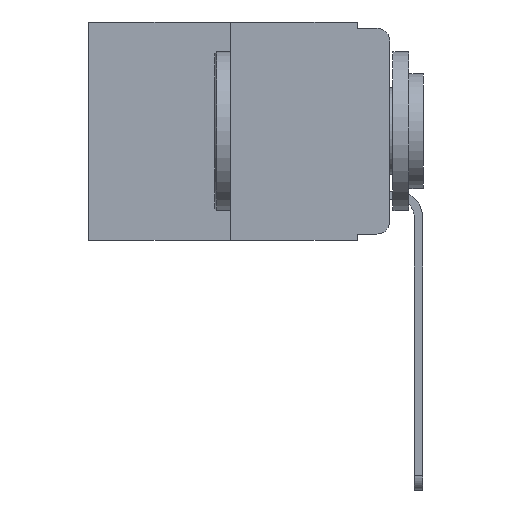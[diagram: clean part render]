
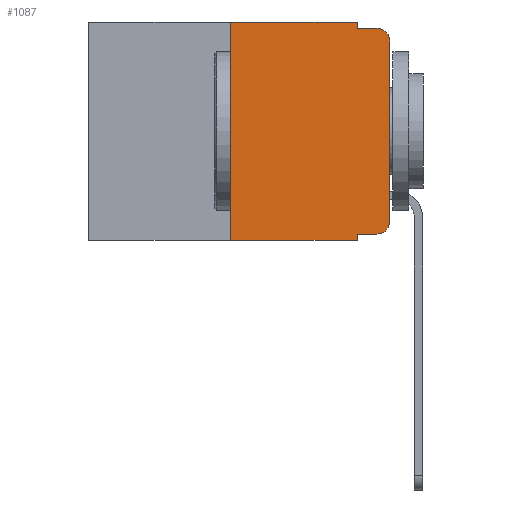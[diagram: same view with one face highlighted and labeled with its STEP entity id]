
A CAD part, left-side view. The second image highlights one B-rep face of the part: STEP entity #1087.
In plain terms, the highlighted planar face has unit normal (-1, 0, 0).
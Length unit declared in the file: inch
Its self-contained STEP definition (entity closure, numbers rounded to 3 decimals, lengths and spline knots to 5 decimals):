
#25 = VERTEX_POINT ( 'NONE', #7749 ) ;
#198 = ORIENTED_EDGE ( 'NONE', *, *, #9880, .T. ) ;
#398 = VERTEX_POINT ( 'NONE', #7649 ) ;
#482 = EDGE_CURVE ( 'NONE', #6446, #1942, #6358, .T. ) ;
#495 = DIRECTION ( 'NONE',  ( 0., -1., 0. ) ) ;
#609 = DIRECTION ( 'NONE',  ( 0., 0., 1. ) ) ;
#621 = AXIS2_PLACEMENT_3D ( 'NONE', #8059, #11972, #12167 ) ;
#648 = VERTEX_POINT ( 'NONE', #6341 ) ;
#877 = ORIENTED_EDGE ( 'NONE', *, *, #10707, .F. ) ;
#1087 = ADVANCED_FACE ( 'NONE', ( #11623 ), #9713, .F. ) ;
#1224 = DIRECTION ( 'NONE',  ( -1., 0., 0. ) ) ;
#1232 = VERTEX_POINT ( 'NONE', #9295 ) ;
#1382 = VECTOR ( 'NONE', #11126, 39.37008 ) ;
#1524 = EDGE_LOOP ( 'NONE', ( #8616, #7306, #877, #11440, #6873, #10229, #10753, #10109, #198, #8325 ) ) ;
#1886 = VECTOR ( 'NONE', #7356, 39.37008 ) ;
#1942 = VERTEX_POINT ( 'NONE', #2944 ) ;
#2054 = VERTEX_POINT ( 'NONE', #10558 ) ;
#2088 = EDGE_CURVE ( 'NONE', #7814, #1232, #7029, .T. ) ;
#2227 = CARTESIAN_POINT ( 'NONE',  ( 0., 0.051, 0. ) ) ;
#2288 = CARTESIAN_POINT ( 'NONE',  ( 0., 0.25, 0. ) ) ;
#2368 = LINE ( 'NONE', #2288, #9553 ) ;
#2627 = VERTEX_POINT ( 'NONE', #10738 ) ;
#2803 = DIRECTION ( 'NONE',  ( 0., -1., 0. ) ) ;
#2851 = VECTOR ( 'NONE', #4229, 39.37008 ) ;
#2944 = CARTESIAN_POINT ( 'NONE',  ( 0., 0.051, -0.343 ) ) ;
#3024 = EDGE_CURVE ( 'NONE', #2054, #25, #5633, .T. ) ;
#3972 = EDGE_CURVE ( 'NONE', #1232, #648, #7456, .T. ) ;
#4229 = DIRECTION ( 'NONE',  ( 0., 0., -1. ) ) ;
#4371 = CARTESIAN_POINT ( 'NONE',  ( 0., 0.02, -0.333 ) ) ;
#4451 = DIRECTION ( 'NONE',  ( -1., 0., 0. ) ) ;
#4474 = CARTESIAN_POINT ( 'NONE',  ( 0., 0.02, -0.313 ) ) ;
#4587 = EDGE_CURVE ( 'NONE', #398, #2054, #8627, .T. ) ;
#4700 = CARTESIAN_POINT ( 'NONE',  ( 0., 0.051, -0.01 ) ) ;
#5633 = LINE ( 'NONE', #2227, #2851 ) ;
#6057 = VECTOR ( 'NONE', #495, 39.37008 ) ;
#6341 = CARTESIAN_POINT ( 'NONE',  ( 0., 0., -0.03 ) ) ;
#6358 = LINE ( 'NONE', #11688, #6057 ) ;
#6428 = CARTESIAN_POINT ( 'NONE',  ( 0., 0.051, -0.333 ) ) ;
#6446 = VERTEX_POINT ( 'NONE', #8092 ) ;
#6471 = DIRECTION ( 'NONE',  ( 0., 0., -1. ) ) ;
#6512 = CARTESIAN_POINT ( 'NONE',  ( 0., 0.473, 0. ) ) ;
#6873 = ORIENTED_EDGE ( 'NONE', *, *, #4587, .F. ) ;
#6930 = CARTESIAN_POINT ( 'NONE',  ( 0., 0.02, -0.03 ) ) ;
#7029 = CIRCLE ( 'NONE', #8880, 0.02 ) ;
#7306 = ORIENTED_EDGE ( 'NONE', *, *, #8290, .T. ) ;
#7356 = DIRECTION ( 'NONE',  ( 0., -1., 0. ) ) ;
#7456 = LINE ( 'NONE', #10349, #9958 ) ;
#7649 = CARTESIAN_POINT ( 'NONE',  ( 0., 0.25, 0. ) ) ;
#7709 = LINE ( 'NONE', #8105, #12233 ) ;
#7749 = CARTESIAN_POINT ( 'NONE',  ( 0., 0.051, -0.01 ) ) ;
#7814 = VERTEX_POINT ( 'NONE', #4371 ) ;
#7849 = DIRECTION ( 'NONE',  ( 0., 0., -1. ) ) ;
#8059 = CARTESIAN_POINT ( 'NONE',  ( 0., 0.473, 0. ) ) ;
#8092 = CARTESIAN_POINT ( 'NONE',  ( 0., 0.25, -0.343 ) ) ;
#8105 = CARTESIAN_POINT ( 'NONE',  ( 0., 0.051, 0. ) ) ;
#8290 = EDGE_CURVE ( 'NONE', #648, #2627, #8998, .T. ) ;
#8325 = ORIENTED_EDGE ( 'NONE', *, *, #2088, .T. ) ;
#8616 = ORIENTED_EDGE ( 'NONE', *, *, #3972, .T. ) ;
#8627 = LINE ( 'NONE', #6512, #1382 ) ;
#8735 = AXIS2_PLACEMENT_3D ( 'NONE', #6930, #1224, #7849 ) ;
#8839 = DIRECTION ( 'NONE',  ( 0., 0., 1. ) ) ;
#8880 = AXIS2_PLACEMENT_3D ( 'NONE', #4474, #4451, #6471 ) ;
#8998 = CIRCLE ( 'NONE', #8735, 0.02 ) ;
#9082 = DIRECTION ( 'NONE',  ( 0., 0., -1. ) ) ;
#9295 = CARTESIAN_POINT ( 'NONE',  ( 0., 0., -0.313 ) ) ;
#9405 = LINE ( 'NONE', #6428, #1886 ) ;
#9553 = VECTOR ( 'NONE', #8839, 39.37008 ) ;
#9629 = EDGE_CURVE ( 'NONE', #6446, #398, #2368, .T. ) ;
#9713 = PLANE ( 'NONE',  #621 ) ;
#9880 = EDGE_CURVE ( 'NONE', #11284, #7814, #9405, .T. ) ;
#9958 = VECTOR ( 'NONE', #609, 39.37008 ) ;
#10038 = CARTESIAN_POINT ( 'NONE',  ( 0., 0.051, -0.333 ) ) ;
#10109 = ORIENTED_EDGE ( 'NONE', *, *, #11239, .F. ) ;
#10229 = ORIENTED_EDGE ( 'NONE', *, *, #9629, .F. ) ;
#10349 = CARTESIAN_POINT ( 'NONE',  ( 0., 0., 0. ) ) ;
#10558 = CARTESIAN_POINT ( 'NONE',  ( 0., 0.051, 0. ) ) ;
#10707 = EDGE_CURVE ( 'NONE', #25, #2627, #11026, .T. ) ;
#10737 = VECTOR ( 'NONE', #2803, 39.37008 ) ;
#10738 = CARTESIAN_POINT ( 'NONE',  ( 0., 0.02, -0.01 ) ) ;
#10753 = ORIENTED_EDGE ( 'NONE', *, *, #482, .T. ) ;
#11026 = LINE ( 'NONE', #4700, #10737 ) ;
#11126 = DIRECTION ( 'NONE',  ( 0., -1., 0. ) ) ;
#11239 = EDGE_CURVE ( 'NONE', #11284, #1942, #7709, .T. ) ;
#11284 = VERTEX_POINT ( 'NONE', #10038 ) ;
#11440 = ORIENTED_EDGE ( 'NONE', *, *, #3024, .F. ) ;
#11623 = FACE_OUTER_BOUND ( 'NONE', #1524, .T. ) ;
#11688 = CARTESIAN_POINT ( 'NONE',  ( 0., 0.473, -0.343 ) ) ;
#11972 = DIRECTION ( 'NONE',  ( 1., 0., 0. ) ) ;
#12167 = DIRECTION ( 'NONE',  ( 0., 0., -1. ) ) ;
#12233 = VECTOR ( 'NONE', #9082, 39.37008 ) ;
